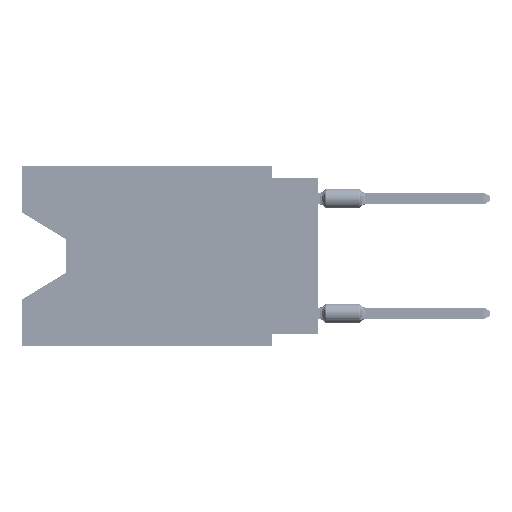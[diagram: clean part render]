
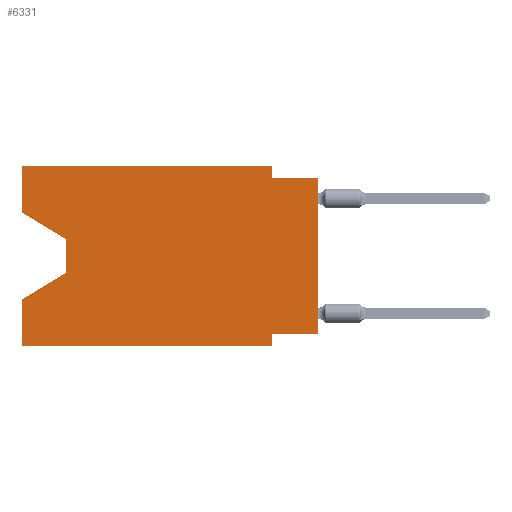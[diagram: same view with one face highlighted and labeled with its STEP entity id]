
A CAD part, left-side view. The second image highlights one B-rep face of the part: STEP entity #6331.
In plain terms, the highlighted planar face has unit normal (-1, 0, 0).
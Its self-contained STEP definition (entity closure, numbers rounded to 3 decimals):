
#269 = CARTESIAN_POINT ( 'NONE',  ( 0., 0., -0.635 ) ) ;
#312 = DIRECTION ( 'NONE',  ( 0., 0., -1. ) ) ;
#317 = LINE ( 'NONE', #659, #57674 ) ;
#445 = EDGE_CURVE ( 'NONE', #58773, #29433, #59323, .T. ) ;
#659 = CARTESIAN_POINT ( 'NONE',  ( 0., 0., -0.635 ) ) ;
#1566 = DIRECTION ( 'NONE',  ( 0., 0., -1. ) ) ;
#1920 = VERTEX_POINT ( 'NONE', #24421 ) ;
#2261 = LINE ( 'NONE', #12050, #36305 ) ;
#3101 = EDGE_CURVE ( 'NONE', #22394, #28374, #44767, .T. ) ;
#3326 = ORIENTED_EDGE ( 'NONE', *, *, #59789, .F. ) ;
#4118 = EDGE_CURVE ( 'NONE', #1920, #26839, #6265, .T. ) ;
#5572 = DIRECTION ( 'NONE',  ( 0., 1., 0. ) ) ;
#6265 = LINE ( 'NONE', #64244, #23796 ) ;
#6331 = ADVANCED_FACE ( 'NONE', ( #17303 ), #38941, .F. ) ;
#6374 = CARTESIAN_POINT ( 'NONE',  ( 0., 16.383, -9.906 ) ) ;
#7302 = VERTEX_POINT ( 'NONE', #67980 ) ;
#7755 = DIRECTION ( 'NONE',  ( 0., -0.855, -0.519 ) ) ;
#7970 = ORIENTED_EDGE ( 'NONE', *, *, #39477, .T. ) ;
#8521 = LINE ( 'NONE', #41013, #55411 ) ;
#9272 = CARTESIAN_POINT ( 'NONE',  ( 0., 16.383, -7.36 ) ) ;
#10422 = ORIENTED_EDGE ( 'NONE', *, *, #4118, .F. ) ;
#10555 = ORIENTED_EDGE ( 'NONE', *, *, #43595, .T. ) ;
#10822 = CARTESIAN_POINT ( 'NONE',  ( 0., 2.54, -9.271 ) ) ;
#11244 = EDGE_CURVE ( 'NONE', #1920, #14142, #67553, .T. ) ;
#11366 = EDGE_CURVE ( 'NONE', #28374, #58773, #49639, .T. ) ;
#12050 = CARTESIAN_POINT ( 'NONE',  ( 0., 13.97, -4.013 ) ) ;
#13158 = VECTOR ( 'NONE', #51165, 1000. ) ;
#13775 = DIRECTION ( 'NONE',  ( 0., 0.855, -0.519 ) ) ;
#14142 = VERTEX_POINT ( 'NONE', #269 ) ;
#14908 = VECTOR ( 'NONE', #36622, 1000. ) ;
#16263 = CARTESIAN_POINT ( 'NONE',  ( 0., 16.383, -2.546 ) ) ;
#17303 = FACE_OUTER_BOUND ( 'NONE', #48869, .T. ) ;
#18506 = ORIENTED_EDGE ( 'NONE', *, *, #27969, .F. ) ;
#19067 = VERTEX_POINT ( 'NONE', #44855 ) ;
#19069 = LINE ( 'NONE', #50479, #13158 ) ;
#19216 = EDGE_CURVE ( 'NONE', #27852, #63746, #8521, .T. ) ;
#19401 = DIRECTION ( 'NONE',  ( 0., 0., 1. ) ) ;
#19926 = EDGE_CURVE ( 'NONE', #62427, #63746, #19069, .T. ) ;
#20715 = VECTOR ( 'NONE', #38522, 1000. ) ;
#20970 = CARTESIAN_POINT ( 'NONE',  ( 0., 2.54, 0. ) ) ;
#22394 = VERTEX_POINT ( 'NONE', #16263 ) ;
#22676 = AXIS2_PLACEMENT_3D ( 'NONE', #45205, #38600, #60217 ) ;
#22823 = CARTESIAN_POINT ( 'NONE',  ( 0., 16.383, -2.546 ) ) ;
#23796 = VECTOR ( 'NONE', #5572, 1000. ) ;
#24421 = CARTESIAN_POINT ( 'NONE',  ( 0., 0., -9.271 ) ) ;
#25165 = ORIENTED_EDGE ( 'NONE', *, *, #11244, .T. ) ;
#26839 = VERTEX_POINT ( 'NONE', #10822 ) ;
#26926 = ORIENTED_EDGE ( 'NONE', *, *, #11366, .F. ) ;
#27029 = ORIENTED_EDGE ( 'NONE', *, *, #19216, .T. ) ;
#27683 = CARTESIAN_POINT ( 'NONE',  ( 0., 16.383, 0. ) ) ;
#27852 = VERTEX_POINT ( 'NONE', #53070 ) ;
#27969 = EDGE_CURVE ( 'NONE', #29433, #14142, #317, .T. ) ;
#28374 = VERTEX_POINT ( 'NONE', #64824 ) ;
#29433 = VERTEX_POINT ( 'NONE', #35249 ) ;
#31044 = LINE ( 'NONE', #31386, #14908 ) ;
#31386 = CARTESIAN_POINT ( 'NONE',  ( 0., 2.54, -9.906 ) ) ;
#32945 = LINE ( 'NONE', #6374, #20715 ) ;
#33608 = DIRECTION ( 'NONE',  ( 0., -1., 0. ) ) ;
#33684 = VECTOR ( 'NONE', #66055, 1000. ) ;
#35249 = CARTESIAN_POINT ( 'NONE',  ( 0., 2.54, -0.635 ) ) ;
#35526 = EDGE_CURVE ( 'NONE', #22394, #7302, #50009, .T. ) ;
#36305 = VECTOR ( 'NONE', #1566, 1000. ) ;
#36533 = VECTOR ( 'NONE', #33608, 1000. ) ;
#36622 = DIRECTION ( 'NONE',  ( 0., 0., -1. ) ) ;
#38522 = DIRECTION ( 'NONE',  ( 0., -1., 0. ) ) ;
#38600 = DIRECTION ( 'NONE',  ( 1., 0., 0. ) ) ;
#38941 = PLANE ( 'NONE',  #22676 ) ;
#39477 = EDGE_CURVE ( 'NONE', #62427, #19067, #32945, .T. ) ;
#40005 = CARTESIAN_POINT ( 'NONE',  ( 0., 0., 0. ) ) ;
#41013 = CARTESIAN_POINT ( 'NONE',  ( 0., 13.97, -5.893 ) ) ;
#43595 = EDGE_CURVE ( 'NONE', #7302, #27852, #2261, .T. ) ;
#44767 = LINE ( 'NONE', #49644, #33684 ) ;
#44855 = CARTESIAN_POINT ( 'NONE',  ( 0., 2.54, -9.906 ) ) ;
#45205 = CARTESIAN_POINT ( 'NONE',  ( 0., 16.383, 0. ) ) ;
#47509 = ORIENTED_EDGE ( 'NONE', *, *, #19926, .F. ) ;
#48869 = EDGE_LOOP ( 'NONE', ( #65496, #10555, #27029, #47509, #7970, #3326, #10422, #25165, #18506, #52078, #26926, #60729 ) ) ;
#49639 = LINE ( 'NONE', #27683, #36533 ) ;
#49644 = CARTESIAN_POINT ( 'NONE',  ( 0., 16.383, 0. ) ) ;
#50009 = LINE ( 'NONE', #22823, #59367 ) ;
#50479 = CARTESIAN_POINT ( 'NONE',  ( 0., 16.383, 0. ) ) ;
#51165 = DIRECTION ( 'NONE',  ( 0., 0., 1. ) ) ;
#52078 = ORIENTED_EDGE ( 'NONE', *, *, #445, .F. ) ;
#53070 = CARTESIAN_POINT ( 'NONE',  ( 0., 13.97, -5.893 ) ) ;
#53148 = CARTESIAN_POINT ( 'NONE',  ( 0., 2.54, 0. ) ) ;
#55411 = VECTOR ( 'NONE', #13775, 1000. ) ;
#56671 = VECTOR ( 'NONE', #312, 1000. ) ;
#57674 = VECTOR ( 'NONE', #64236, 1000. ) ;
#58773 = VERTEX_POINT ( 'NONE', #53148 ) ;
#59323 = LINE ( 'NONE', #20970, #56671 ) ;
#59367 = VECTOR ( 'NONE', #7755, 1000. ) ;
#59789 = EDGE_CURVE ( 'NONE', #26839, #19067, #31044, .T. ) ;
#60217 = DIRECTION ( 'NONE',  ( 0., 0., -1. ) ) ;
#60729 = ORIENTED_EDGE ( 'NONE', *, *, #3101, .F. ) ;
#62427 = VERTEX_POINT ( 'NONE', #64945 ) ;
#63746 = VERTEX_POINT ( 'NONE', #9272 ) ;
#64236 = DIRECTION ( 'NONE',  ( 0., -1., 0. ) ) ;
#64244 = CARTESIAN_POINT ( 'NONE',  ( 0., 0., -9.271 ) ) ;
#64824 = CARTESIAN_POINT ( 'NONE',  ( 0., 16.383, 0. ) ) ;
#64945 = CARTESIAN_POINT ( 'NONE',  ( 0., 16.383, -9.906 ) ) ;
#65496 = ORIENTED_EDGE ( 'NONE', *, *, #35526, .T. ) ;
#66055 = DIRECTION ( 'NONE',  ( 0., 0., 1. ) ) ;
#67553 = LINE ( 'NONE', #40005, #67718 ) ;
#67718 = VECTOR ( 'NONE', #19401, 1000. ) ;
#67980 = CARTESIAN_POINT ( 'NONE',  ( 0., 13.97, -4.013 ) ) ;
